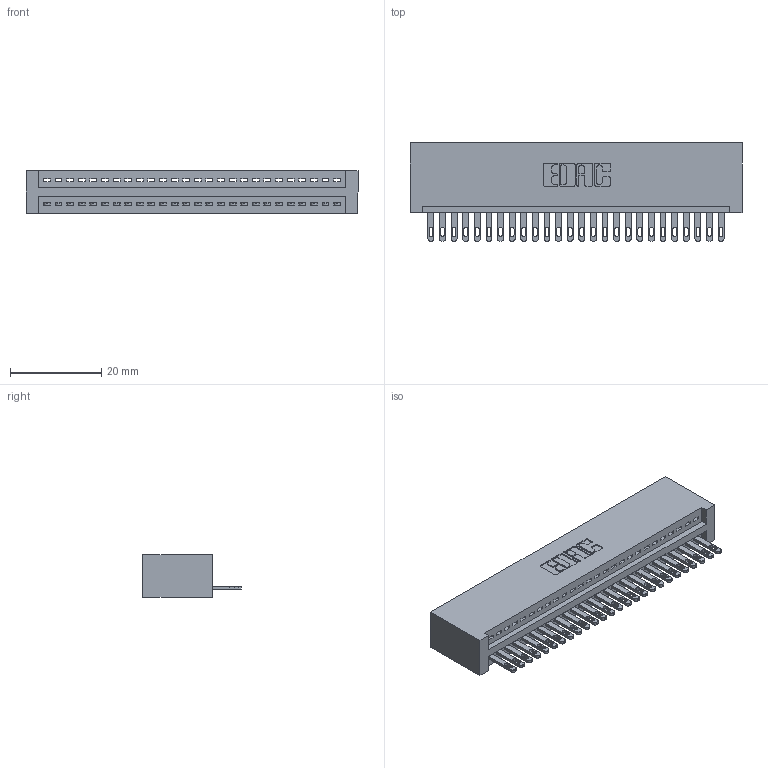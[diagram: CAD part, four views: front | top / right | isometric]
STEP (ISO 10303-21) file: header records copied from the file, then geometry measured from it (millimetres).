
FILE_DESCRIPTION (( 'STEP AP203' ), '1' );
FILE_NAME ('345-026-500-101.STEP', '2019-10-07T01:29:50', ( '' ), ( '' ), 'SwSTEP 2.0', 'SolidWorks 2016', '' );
FILE_SCHEMA (( 'CONFIG_CONTROL_DESIGN' ));
Length unit declared in the file: inch
Products named in the file (3): 345-292-001_345-293-100; 345 Part_No Mounting Lugs; 345-026-500-101
Assembly tree (27 placements, depth 2):
  345-026-500-101
    345 Part_No Mounting Lugs
    345-292-001_345-293-100  x26
Bounding box: 72.64 x 21.51 x 9.4 mm (x, y, z)
Volume: 7369.2 mm3; surface area: 9824.1 mm2
Topology: 27 solids, 27 shells, 1522 faces, 4685 edges, 3122 vertices
Faces by surface type: plane 960, cylinder 562
Entity records: 21375 total; most frequent: CARTESIAN_POINT 3710, ORIENTED_EDGE 3670, DIRECTION 3259, EDGE_CURVE 1835, LINE 1603, VECTOR 1603, VERTEX_POINT 1222, AXIS2_PLACEMENT_3D 828
